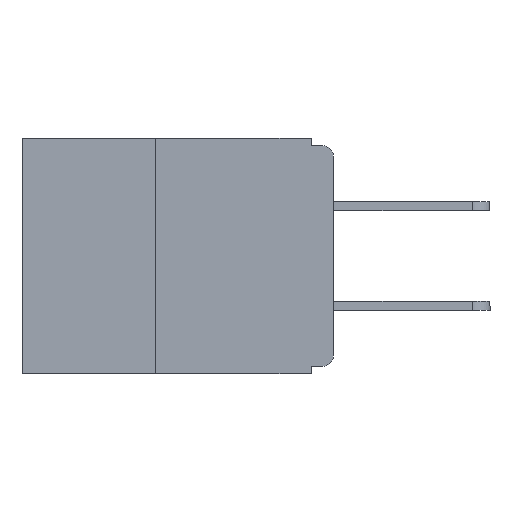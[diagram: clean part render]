
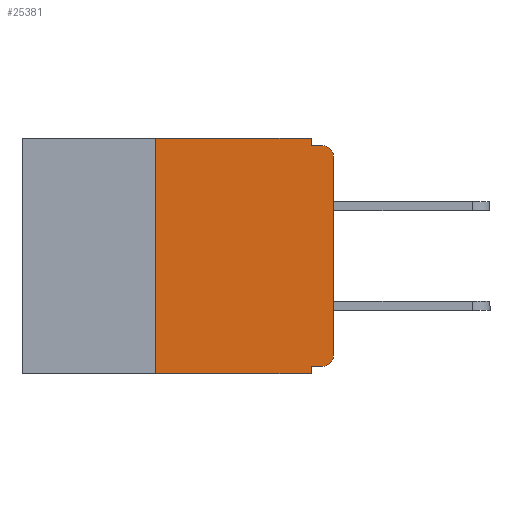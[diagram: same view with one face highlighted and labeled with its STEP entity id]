
A CAD part, left-side view. The second image highlights one B-rep face of the part: STEP entity #25381.
In plain terms, the highlighted planar face has unit normal (-1, 0, 0).
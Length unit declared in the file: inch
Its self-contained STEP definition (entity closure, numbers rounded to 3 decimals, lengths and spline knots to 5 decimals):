
#72 = CARTESIAN_POINT ( 'NONE',  ( 0., 0.437, 0. ) ) ;
#105 = VERTEX_POINT ( 'NONE', #2190 ) ;
#1234 = EDGE_CURVE ( 'NONE', #6632, #105, #17373, .T. ) ;
#1500 = CARTESIAN_POINT ( 'NONE',  ( 0., 0.437, 0. ) ) ;
#2003 = CARTESIAN_POINT ( 'NONE',  ( 0., 0., -0.01 ) ) ;
#2190 = CARTESIAN_POINT ( 'NONE',  ( 0., 0.031, -0.33 ) ) ;
#3205 = AXIS2_PLACEMENT_3D ( 'NONE', #12802, #30810, #15424 ) ;
#3702 = LINE ( 'NONE', #27318, #4538 ) ;
#3983 = CIRCLE ( 'NONE', #24837, 0.015 ) ;
#4179 = DIRECTION ( 'NONE',  ( 1., 0., 0. ) ) ;
#4345 = DIRECTION ( 'NONE',  ( -1., 0., 0. ) ) ;
#4538 = VECTOR ( 'NONE', #9217, 39.37008 ) ;
#4694 = DIRECTION ( 'NONE',  ( 0., -1., 0. ) ) ;
#4757 = ORIENTED_EDGE ( 'NONE', *, *, #28298, .F. ) ;
#4775 = EDGE_CURVE ( 'NONE', #15195, #14522, #12323, .T. ) ;
#5272 = VECTOR ( 'NONE', #16098, 39.37008 ) ;
#5618 = ORIENTED_EDGE ( 'NONE', *, *, #30481, .T. ) ;
#6538 = AXIS2_PLACEMENT_3D ( 'NONE', #1500, #4179, #22534 ) ;
#6632 = VERTEX_POINT ( 'NONE', #8084 ) ;
#6712 = ORIENTED_EDGE ( 'NONE', *, *, #25945, .T. ) ;
#6974 = VECTOR ( 'NONE', #32667, 39.37008 ) ;
#8084 = CARTESIAN_POINT ( 'NONE',  ( 0., 0.031, -0.32 ) ) ;
#8361 = CARTESIAN_POINT ( 'NONE',  ( 0., 0.015, -0.01 ) ) ;
#8424 = LINE ( 'NONE', #2003, #9268 ) ;
#8512 = VERTEX_POINT ( 'NONE', #14709 ) ;
#9217 = DIRECTION ( 'NONE',  ( 0., 0., 1. ) ) ;
#9268 = VECTOR ( 'NONE', #4694, 39.37008 ) ;
#9294 = CARTESIAN_POINT ( 'NONE',  ( 0., 0.25, 0. ) ) ;
#9307 = CIRCLE ( 'NONE', #3205, 0.015 ) ;
#9476 = PLANE ( 'NONE',  #6538 ) ;
#10475 = VECTOR ( 'NONE', #28909, 39.37008 ) ;
#10529 = EDGE_CURVE ( 'NONE', #14086, #24649, #8424, .T. ) ;
#10698 = LINE ( 'NONE', #28990, #16796 ) ;
#11951 = VERTEX_POINT ( 'NONE', #28664 ) ;
#12323 = LINE ( 'NONE', #72, #5272 ) ;
#12802 = CARTESIAN_POINT ( 'NONE',  ( 0., 0.015, -0.305 ) ) ;
#13363 = ORIENTED_EDGE ( 'NONE', *, *, #10529, .F. ) ;
#13966 = LINE ( 'NONE', #30161, #6974 ) ;
#14086 = VERTEX_POINT ( 'NONE', #25576 ) ;
#14522 = VERTEX_POINT ( 'NONE', #17072 ) ;
#14573 = CARTESIAN_POINT ( 'NONE',  ( 0., 0., -0.305 ) ) ;
#14709 = CARTESIAN_POINT ( 'NONE',  ( 0., 0., -0.025 ) ) ;
#14751 = ORIENTED_EDGE ( 'NONE', *, *, #27181, .F. ) ;
#15195 = VERTEX_POINT ( 'NONE', #9294 ) ;
#15424 = DIRECTION ( 'NONE',  ( 0., 0., -1. ) ) ;
#16098 = DIRECTION ( 'NONE',  ( 0., -1., 0. ) ) ;
#16142 = DIRECTION ( 'NONE',  ( 0., 1., 0. ) ) ;
#16429 = ORIENTED_EDGE ( 'NONE', *, *, #1234, .F. ) ;
#16435 = ORIENTED_EDGE ( 'NONE', *, *, #18595, .F. ) ;
#16796 = VECTOR ( 'NONE', #16142, 39.37008 ) ;
#17072 = CARTESIAN_POINT ( 'NONE',  ( 0., 0.031, 0. ) ) ;
#17373 = LINE ( 'NONE', #28942, #10475 ) ;
#18595 = EDGE_CURVE ( 'NONE', #30175, #15195, #21591, .T. ) ;
#18740 = CARTESIAN_POINT ( 'NONE',  ( 0., 0.25, -0.33 ) ) ;
#18897 = VECTOR ( 'NONE', #24559, 39.37008 ) ;
#19479 = CARTESIAN_POINT ( 'NONE',  ( 0., 0.031, 0. ) ) ;
#19506 = ORIENTED_EDGE ( 'NONE', *, *, #24323, .T. ) ;
#19664 = EDGE_LOOP ( 'NONE', ( #6712, #19506, #13363, #14751, #30679, #16435, #5618, #16429, #4757, #22230 ) ) ;
#19890 = EDGE_CURVE ( 'NONE', #11951, #25971, #9307, .T. ) ;
#20116 = CARTESIAN_POINT ( 'NONE',  ( 0., 0.015, -0.025 ) ) ;
#21208 = CARTESIAN_POINT ( 'NONE',  ( 0., 0.25, -0.33 ) ) ;
#21591 = LINE ( 'NONE', #18740, #32748 ) ;
#22230 = ORIENTED_EDGE ( 'NONE', *, *, #19890, .T. ) ;
#22534 = DIRECTION ( 'NONE',  ( 0., 0., -1. ) ) ;
#22711 = DIRECTION ( 'NONE',  ( 0., 0., -1. ) ) ;
#23918 = DIRECTION ( 'NONE',  ( 0., 0., 1. ) ) ;
#24323 = EDGE_CURVE ( 'NONE', #8512, #24649, #3983, .T. ) ;
#24559 = DIRECTION ( 'NONE',  ( 0., 0., -1. ) ) ;
#24649 = VERTEX_POINT ( 'NONE', #8361 ) ;
#24837 = AXIS2_PLACEMENT_3D ( 'NONE', #20116, #4345, #22711 ) ;
#25381 = ADVANCED_FACE ( 'NONE', ( #28650 ), #9476, .F. ) ;
#25576 = CARTESIAN_POINT ( 'NONE',  ( 0., 0.031, -0.01 ) ) ;
#25945 = EDGE_CURVE ( 'NONE', #25971, #8512, #3702, .T. ) ;
#25971 = VERTEX_POINT ( 'NONE', #14573 ) ;
#26558 = LINE ( 'NONE', #19479, #18897 ) ;
#27181 = EDGE_CURVE ( 'NONE', #14522, #14086, #26558, .T. ) ;
#27318 = CARTESIAN_POINT ( 'NONE',  ( 0., 0., 0. ) ) ;
#28298 = EDGE_CURVE ( 'NONE', #11951, #6632, #10698, .T. ) ;
#28650 = FACE_OUTER_BOUND ( 'NONE', #19664, .T. ) ;
#28664 = CARTESIAN_POINT ( 'NONE',  ( 0., 0.015, -0.32 ) ) ;
#28909 = DIRECTION ( 'NONE',  ( 0., 0., -1. ) ) ;
#28942 = CARTESIAN_POINT ( 'NONE',  ( 0., 0.031, -0.33 ) ) ;
#28990 = CARTESIAN_POINT ( 'NONE',  ( 0., 0., -0.32 ) ) ;
#30161 = CARTESIAN_POINT ( 'NONE',  ( 0., 0.437, -0.33 ) ) ;
#30175 = VERTEX_POINT ( 'NONE', #21208 ) ;
#30481 = EDGE_CURVE ( 'NONE', #30175, #105, #13966, .T. ) ;
#30679 = ORIENTED_EDGE ( 'NONE', *, *, #4775, .F. ) ;
#30810 = DIRECTION ( 'NONE',  ( -1., 0., 0. ) ) ;
#32667 = DIRECTION ( 'NONE',  ( 0., -1., 0. ) ) ;
#32748 = VECTOR ( 'NONE', #23918, 39.37008 ) ;
